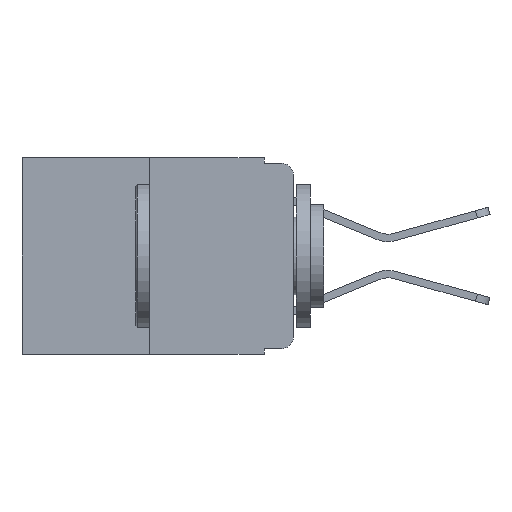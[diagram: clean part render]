
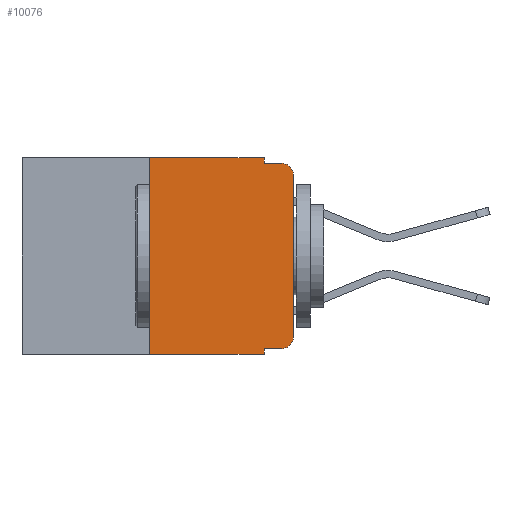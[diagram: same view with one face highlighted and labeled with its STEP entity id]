
A CAD part, left-side view. The second image highlights one B-rep face of the part: STEP entity #10076.
In plain terms, the highlighted planar face has unit normal (-1, 0, 0).
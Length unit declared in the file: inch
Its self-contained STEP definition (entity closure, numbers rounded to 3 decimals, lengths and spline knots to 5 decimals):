
#13 = CARTESIAN_POINT ( 'NONE',  ( 0., 0.473, 0. ) ) ;
#115 = EDGE_CURVE ( 'NONE', #3008, #7521, #11538, .T. ) ;
#250 = CARTESIAN_POINT ( 'NONE',  ( 0., 0., -0.03 ) ) ;
#584 = EDGE_CURVE ( 'NONE', #1362, #8008, #8659, .T. ) ;
#761 = CARTESIAN_POINT ( 'NONE',  ( 0., 0.25, 0. ) ) ;
#826 = AXIS2_PLACEMENT_3D ( 'NONE', #12330, #10443, #4697 ) ;
#930 = VECTOR ( 'NONE', #9278, 39.37008 ) ;
#1075 = CARTESIAN_POINT ( 'NONE',  ( 0., 0.051, -0.333 ) ) ;
#1115 = DIRECTION ( 'NONE',  ( 0., 0., -1. ) ) ;
#1194 = DIRECTION ( 'NONE',  ( 0., 0., -1. ) ) ;
#1309 = CARTESIAN_POINT ( 'NONE',  ( 0., 0.051, -0.333 ) ) ;
#1319 = VERTEX_POINT ( 'NONE', #10989 ) ;
#1362 = VERTEX_POINT ( 'NONE', #8122 ) ;
#1443 = CARTESIAN_POINT ( 'NONE',  ( 0., 0., 0. ) ) ;
#1698 = DIRECTION ( 'NONE',  ( 0., 0., -1. ) ) ;
#1951 = PLANE ( 'NONE',  #2144 ) ;
#2009 = EDGE_CURVE ( 'NONE', #8008, #11484, #5089, .T. ) ;
#2030 = DIRECTION ( 'NONE',  ( 0., -1., 0. ) ) ;
#2144 = AXIS2_PLACEMENT_3D ( 'NONE', #12301, #2718, #1698 ) ;
#2468 = DIRECTION ( 'NONE',  ( 0., 0., 1. ) ) ;
#2476 = CARTESIAN_POINT ( 'NONE',  ( 0., 0.473, -0.343 ) ) ;
#2602 = LINE ( 'NONE', #2476, #9561 ) ;
#2652 = CIRCLE ( 'NONE', #826, 0.02 ) ;
#2718 = DIRECTION ( 'NONE',  ( 1., 0., 0. ) ) ;
#3008 = VERTEX_POINT ( 'NONE', #1309 ) ;
#3069 = VERTEX_POINT ( 'NONE', #5916 ) ;
#3149 = VECTOR ( 'NONE', #11522, 39.37008 ) ;
#3182 = ORIENTED_EDGE ( 'NONE', *, *, #10801, .F. ) ;
#3202 = VECTOR ( 'NONE', #11784, 39.37008 ) ;
#3466 = CARTESIAN_POINT ( 'NONE',  ( 0., 0.02, -0.333 ) ) ;
#3647 = CIRCLE ( 'NONE', #10716, 0.02 ) ;
#3712 = VECTOR ( 'NONE', #3876, 39.37008 ) ;
#3756 = EDGE_CURVE ( 'NONE', #3907, #11484, #2652, .T. ) ;
#3876 = DIRECTION ( 'NONE',  ( 0., -1., 0. ) ) ;
#3907 = VERTEX_POINT ( 'NONE', #250 ) ;
#4323 = EDGE_CURVE ( 'NONE', #11191, #6697, #3647, .T. ) ;
#4361 = EDGE_CURVE ( 'NONE', #3008, #11191, #10737, .T. ) ;
#4495 = ORIENTED_EDGE ( 'NONE', *, *, #4590, .T. ) ;
#4590 = EDGE_CURVE ( 'NONE', #6697, #3907, #6241, .T. ) ;
#4697 = DIRECTION ( 'NONE',  ( 0., 0., -1. ) ) ;
#5089 = LINE ( 'NONE', #9943, #3202 ) ;
#5171 = ORIENTED_EDGE ( 'NONE', *, *, #2009, .F. ) ;
#5278 = VECTOR ( 'NONE', #2030, 39.37008 ) ;
#5400 = EDGE_LOOP ( 'NONE', ( #4495, #9896, #5171, #9251, #7473, #3182, #9765, #8078, #6935, #6963 ) ) ;
#5916 = CARTESIAN_POINT ( 'NONE',  ( 0., 0.25, -0.343 ) ) ;
#5999 = DIRECTION ( 'NONE',  ( -1., 0., 0. ) ) ;
#6241 = LINE ( 'NONE', #1443, #10723 ) ;
#6316 = DIRECTION ( 'NONE',  ( 0., -1., 0. ) ) ;
#6697 = VERTEX_POINT ( 'NONE', #8664 ) ;
#6749 = FACE_OUTER_BOUND ( 'NONE', #5400, .T. ) ;
#6789 = LINE ( 'NONE', #13, #3712 ) ;
#6935 = ORIENTED_EDGE ( 'NONE', *, *, #4361, .T. ) ;
#6963 = ORIENTED_EDGE ( 'NONE', *, *, #4323, .T. ) ;
#7137 = CARTESIAN_POINT ( 'NONE',  ( 0., 0.02, -0.01 ) ) ;
#7432 = LINE ( 'NONE', #761, #930 ) ;
#7473 = ORIENTED_EDGE ( 'NONE', *, *, #8693, .F. ) ;
#7521 = VERTEX_POINT ( 'NONE', #10759 ) ;
#7660 = CARTESIAN_POINT ( 'NONE',  ( 0., 0.051, 0. ) ) ;
#8008 = VERTEX_POINT ( 'NONE', #8888 ) ;
#8078 = ORIENTED_EDGE ( 'NONE', *, *, #115, .F. ) ;
#8112 = EDGE_CURVE ( 'NONE', #3069, #7521, #2602, .T. ) ;
#8122 = CARTESIAN_POINT ( 'NONE',  ( 0., 0.051, 0. ) ) ;
#8551 = CARTESIAN_POINT ( 'NONE',  ( 0., 0.051, 0. ) ) ;
#8659 = LINE ( 'NONE', #7660, #3149 ) ;
#8664 = CARTESIAN_POINT ( 'NONE',  ( 0., 0., -0.313 ) ) ;
#8693 = EDGE_CURVE ( 'NONE', #1319, #1362, #6789, .T. ) ;
#8888 = CARTESIAN_POINT ( 'NONE',  ( 0., 0.051, -0.01 ) ) ;
#9251 = ORIENTED_EDGE ( 'NONE', *, *, #584, .F. ) ;
#9278 = DIRECTION ( 'NONE',  ( 0., 0., 1. ) ) ;
#9561 = VECTOR ( 'NONE', #6316, 39.37008 ) ;
#9724 = CARTESIAN_POINT ( 'NONE',  ( 0., 0.02, -0.313 ) ) ;
#9765 = ORIENTED_EDGE ( 'NONE', *, *, #8112, .T. ) ;
#9896 = ORIENTED_EDGE ( 'NONE', *, *, #3756, .T. ) ;
#9943 = CARTESIAN_POINT ( 'NONE',  ( 0., 0.051, -0.01 ) ) ;
#10076 = ADVANCED_FACE ( 'NONE', ( #6749 ), #1951, .F. ) ;
#10443 = DIRECTION ( 'NONE',  ( -1., 0., 0. ) ) ;
#10657 = VECTOR ( 'NONE', #1115, 39.37008 ) ;
#10716 = AXIS2_PLACEMENT_3D ( 'NONE', #9724, #5999, #1194 ) ;
#10723 = VECTOR ( 'NONE', #2468, 39.37008 ) ;
#10737 = LINE ( 'NONE', #1075, #5278 ) ;
#10759 = CARTESIAN_POINT ( 'NONE',  ( 0., 0.051, -0.343 ) ) ;
#10801 = EDGE_CURVE ( 'NONE', #3069, #1319, #7432, .T. ) ;
#10989 = CARTESIAN_POINT ( 'NONE',  ( 0., 0.25, 0. ) ) ;
#11191 = VERTEX_POINT ( 'NONE', #3466 ) ;
#11484 = VERTEX_POINT ( 'NONE', #7137 ) ;
#11522 = DIRECTION ( 'NONE',  ( 0., 0., -1. ) ) ;
#11538 = LINE ( 'NONE', #8551, #10657 ) ;
#11784 = DIRECTION ( 'NONE',  ( 0., -1., 0. ) ) ;
#12301 = CARTESIAN_POINT ( 'NONE',  ( 0., 0.473, 0. ) ) ;
#12330 = CARTESIAN_POINT ( 'NONE',  ( 0., 0.02, -0.03 ) ) ;
